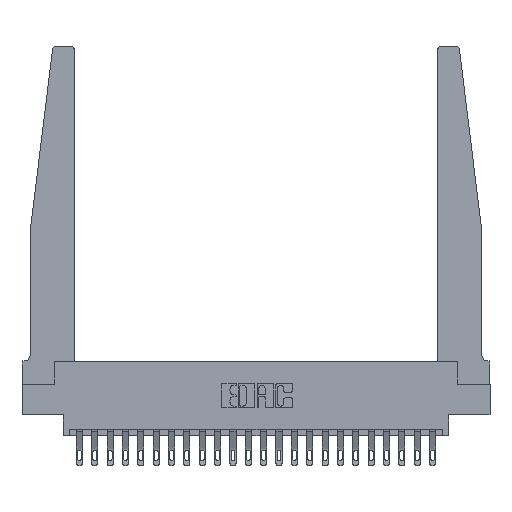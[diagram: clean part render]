
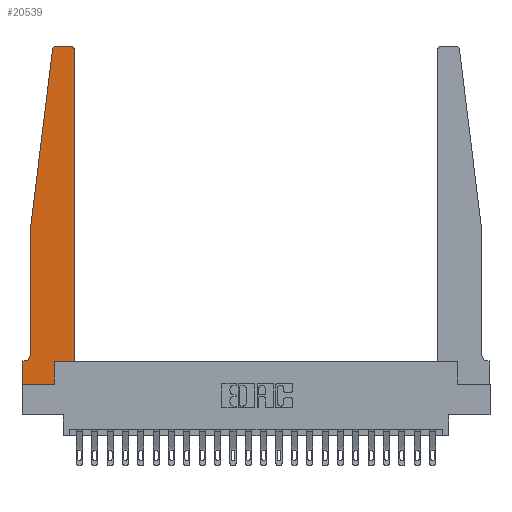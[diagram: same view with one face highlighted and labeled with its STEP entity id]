
A CAD part, top view. The second image highlights one B-rep face of the part: STEP entity #20539.
In plain terms, the highlighted planar face has unit normal (0, 0, 1).
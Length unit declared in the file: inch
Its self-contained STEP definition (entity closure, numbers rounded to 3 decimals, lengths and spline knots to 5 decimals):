
#164 = VERTEX_POINT ( 'NONE', #22766 ) ;
#197 = VERTEX_POINT ( 'NONE', #15202 ) ;
#421 = CARTESIAN_POINT ( 'NONE',  ( 0.395, 2.72, 0.37 ) ) ;
#449 = LINE ( 'NONE', #17853, #13325 ) ;
#764 = LINE ( 'NONE', #6170, #6350 ) ;
#812 = LINE ( 'NONE', #11622, #9129 ) ;
#1824 = LINE ( 'NONE', #3641, #22793 ) ;
#1828 = VERTEX_POINT ( 'NONE', #13379 ) ;
#1953 = CARTESIAN_POINT ( 'NONE',  ( 0.27653, 2.75, 0.37 ) ) ;
#2102 = CARTESIAN_POINT ( 'NONE',  ( 0., 0.1875, 0.37 ) ) ;
#2241 = VERTEX_POINT ( 'NONE', #5914 ) ;
#2633 = VECTOR ( 'NONE', #14625, 39.37008 ) ;
#3345 = EDGE_CURVE ( 'NONE', #17804, #2241, #1824, .T. ) ;
#3411 = AXIS2_PLACEMENT_3D ( 'NONE', #421, #16656, #18335 ) ;
#3421 = VECTOR ( 'NONE', #14373, 39.37008 ) ;
#3432 = CIRCLE ( 'NONE', #22256, 0.03 ) ;
#3641 = CARTESIAN_POINT ( 'NONE',  ( 0.065, 1.25, 0.37 ) ) ;
#3664 = CARTESIAN_POINT ( 'NONE',  ( 0.425, 0.18, 0.37 ) ) ;
#3665 = ORIENTED_EDGE ( 'NONE', *, *, #15330, .T. ) ;
#3667 = DIRECTION ( 'NONE',  ( 0., 0., -1. ) ) ;
#3907 = LINE ( 'NONE', #12912, #9916 ) ;
#5259 = ORIENTED_EDGE ( 'NONE', *, *, #21274, .T. ) ;
#5590 = LINE ( 'NONE', #23511, #3421 ) ;
#5914 = CARTESIAN_POINT ( 'NONE',  ( 0.065, 0.2375, 0.37 ) ) ;
#5980 = DIRECTION ( 'NONE',  ( 1., 0., 0. ) ) ;
#6170 = CARTESIAN_POINT ( 'NONE',  ( 0.2605, 0.18, 0.37 ) ) ;
#6350 = VECTOR ( 'NONE', #8272, 39.37008 ) ;
#6449 = ORIENTED_EDGE ( 'NONE', *, *, #10601, .T. ) ;
#6654 = ORIENTED_EDGE ( 'NONE', *, *, #22472, .T. ) ;
#6925 = VERTEX_POINT ( 'NONE', #7494 ) ;
#7494 = CARTESIAN_POINT ( 'NONE',  ( 0.395, 2.75, 0.37 ) ) ;
#7627 = DIRECTION ( 'NONE',  ( 0., 0., 1. ) ) ;
#7791 = LINE ( 'NONE', #15153, #14126 ) ;
#8101 = DIRECTION ( 'NONE',  ( -1., 0., 0. ) ) ;
#8272 = DIRECTION ( 'NONE',  ( 0., 1., 0. ) ) ;
#8309 = DIRECTION ( 'NONE',  ( 0., -1., 0. ) ) ;
#8410 = VERTEX_POINT ( 'NONE', #23372 ) ;
#8716 = EDGE_CURVE ( 'NONE', #8410, #197, #764, .T. ) ;
#9026 = DIRECTION ( 'NONE',  ( 0., -1., 0. ) ) ;
#9129 = VECTOR ( 'NONE', #8101, 39.37008 ) ;
#9181 = DIRECTION ( 'NONE',  ( 1., 0., 0. ) ) ;
#9381 = CARTESIAN_POINT ( 'NONE',  ( 0.065, 1.25, 0.37 ) ) ;
#9416 = DIRECTION ( 'NONE',  ( 0., 0., 1. ) ) ;
#9473 = EDGE_CURVE ( 'NONE', #12084, #17281, #449, .T. ) ;
#9916 = VECTOR ( 'NONE', #9181, 39.37008 ) ;
#9934 = VECTOR ( 'NONE', #5980, 39.37008 ) ;
#9944 = CIRCLE ( 'NONE', #21087, 0.05 ) ;
#10035 = CARTESIAN_POINT ( 'NONE',  ( 0.425, 0.18, 0.37 ) ) ;
#10601 = EDGE_CURVE ( 'NONE', #6925, #14703, #7791, .T. ) ;
#10980 = DIRECTION ( 'NONE',  ( -1., 0., 0. ) ) ;
#11041 = ORIENTED_EDGE ( 'NONE', *, *, #22468, .T. ) ;
#11113 = ORIENTED_EDGE ( 'NONE', *, *, #15445, .T. ) ;
#11208 = ORIENTED_EDGE ( 'NONE', *, *, #12326, .T. ) ;
#11236 = FACE_OUTER_BOUND ( 'NONE', #11933, .T. ) ;
#11320 = ORIENTED_EDGE ( 'NONE', *, *, #9473, .T. ) ;
#11622 = CARTESIAN_POINT ( 'NONE',  ( 0.065, 0.1875, 0.37 ) ) ;
#11842 = CIRCLE ( 'NONE', #3411, 0.03 ) ;
#11933 = EDGE_LOOP ( 'NONE', ( #6449, #11208, #3665, #14359, #11113, #5259, #11320, #6654, #23236, #20916, #15470, #11041 ) ) ;
#12084 = VERTEX_POINT ( 'NONE', #13442 ) ;
#12326 = EDGE_CURVE ( 'NONE', #14703, #1828, #3432, .T. ) ;
#12912 = CARTESIAN_POINT ( 'NONE',  ( 0., 0., 0.37 ) ) ;
#13325 = VECTOR ( 'NONE', #8309, 39.37008 ) ;
#13379 = CARTESIAN_POINT ( 'NONE',  ( 0.24675, 2.72367, 0.37 ) ) ;
#13442 = CARTESIAN_POINT ( 'NONE',  ( 0., 0.1875, 0.37 ) ) ;
#13671 = EDGE_CURVE ( 'NONE', #197, #16951, #20528, .T. ) ;
#14126 = VECTOR ( 'NONE', #20685, 39.37008 ) ;
#14359 = ORIENTED_EDGE ( 'NONE', *, *, #3345, .T. ) ;
#14373 = DIRECTION ( 'NONE',  ( -0.122, -0.992, 0. ) ) ;
#14514 = CARTESIAN_POINT ( 'NONE',  ( 0.27653, 2.72, 0.37 ) ) ;
#14625 = DIRECTION ( 'NONE',  ( 0., 1., 0. ) ) ;
#14703 = VERTEX_POINT ( 'NONE', #1953 ) ;
#14987 = DIRECTION ( 'NONE',  ( 1., 0., 0. ) ) ;
#15129 = CARTESIAN_POINT ( 'NONE',  ( 0.425, 0.18, 0.37 ) ) ;
#15153 = CARTESIAN_POINT ( 'NONE',  ( 0.25, 2.75, 0.37 ) ) ;
#15202 = CARTESIAN_POINT ( 'NONE',  ( 0.2605, 0.18, 0.37 ) ) ;
#15330 = EDGE_CURVE ( 'NONE', #1828, #17804, #5590, .T. ) ;
#15375 = VERTEX_POINT ( 'NONE', #16410 ) ;
#15445 = EDGE_CURVE ( 'NONE', #2241, #15375, #9944, .T. ) ;
#15470 = ORIENTED_EDGE ( 'NONE', *, *, #22450, .T. ) ;
#15665 = AXIS2_PLACEMENT_3D ( 'NONE', #2102, #9416, #14987 ) ;
#16410 = CARTESIAN_POINT ( 'NONE',  ( 0.015, 0.1875, 0.37 ) ) ;
#16656 = DIRECTION ( 'NONE',  ( 0., 0., 1. ) ) ;
#16951 = VERTEX_POINT ( 'NONE', #10035 ) ;
#17281 = VERTEX_POINT ( 'NONE', #20715 ) ;
#17804 = VERTEX_POINT ( 'NONE', #9381 ) ;
#17853 = CARTESIAN_POINT ( 'NONE',  ( 0., 0., 0.37 ) ) ;
#18335 = DIRECTION ( 'NONE',  ( 1., 0., 0. ) ) ;
#18595 = PLANE ( 'NONE',  #15665 ) ;
#20141 = CARTESIAN_POINT ( 'NONE',  ( 0.015, 0.2375, 0.37 ) ) ;
#20528 = LINE ( 'NONE', #15129, #9934 ) ;
#20539 = ADVANCED_FACE ( 'NONE', ( #11236 ), #18595, .T. ) ;
#20685 = DIRECTION ( 'NONE',  ( -1., 0., 0. ) ) ;
#20715 = CARTESIAN_POINT ( 'NONE',  ( 0., 0., 0.37 ) ) ;
#20916 = ORIENTED_EDGE ( 'NONE', *, *, #13671, .T. ) ;
#21087 = AXIS2_PLACEMENT_3D ( 'NONE', #20141, #3667, #10980 ) ;
#21274 = EDGE_CURVE ( 'NONE', #15375, #12084, #812, .T. ) ;
#22256 = AXIS2_PLACEMENT_3D ( 'NONE', #14514, #7627, #23648 ) ;
#22450 = EDGE_CURVE ( 'NONE', #16951, #164, #23745, .T. ) ;
#22468 = EDGE_CURVE ( 'NONE', #164, #6925, #11842, .T. ) ;
#22472 = EDGE_CURVE ( 'NONE', #17281, #8410, #3907, .T. ) ;
#22766 = CARTESIAN_POINT ( 'NONE',  ( 0.425, 2.72, 0.37 ) ) ;
#22793 = VECTOR ( 'NONE', #9026, 39.37008 ) ;
#23236 = ORIENTED_EDGE ( 'NONE', *, *, #8716, .T. ) ;
#23372 = CARTESIAN_POINT ( 'NONE',  ( 0.2605, 0., 0.37 ) ) ;
#23511 = CARTESIAN_POINT ( 'NONE',  ( 0.065, 1.25, 0.37 ) ) ;
#23648 = DIRECTION ( 'NONE',  ( 1., 0., 0. ) ) ;
#23745 = LINE ( 'NONE', #3664, #2633 ) ;
